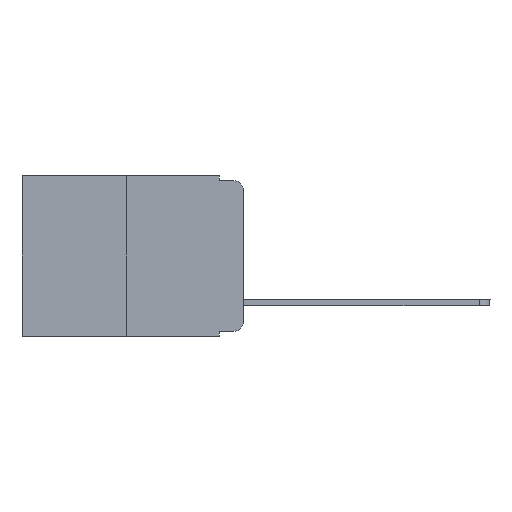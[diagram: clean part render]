
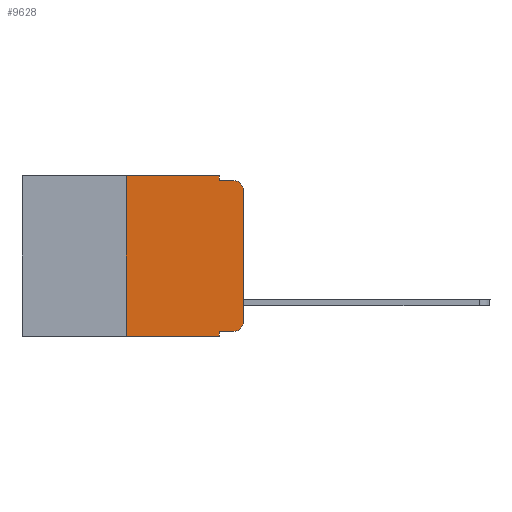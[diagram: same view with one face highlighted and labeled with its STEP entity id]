
A CAD part, left-side view. The second image highlights one B-rep face of the part: STEP entity #9628.
In plain terms, the highlighted planar face has unit normal (-1, 0, 0).
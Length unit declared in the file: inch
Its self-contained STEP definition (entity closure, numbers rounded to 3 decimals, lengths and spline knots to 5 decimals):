
#11 = EDGE_CURVE ( 'NONE', #8862, #13392, #11300, .T. ) ;
#152 = ORIENTED_EDGE ( 'NONE', *, *, #3422, .T. ) ;
#345 = EDGE_CURVE ( 'NONE', #2818, #1427, #13647, .T. ) ;
#547 = VERTEX_POINT ( 'NONE', #5646 ) ;
#638 = CARTESIAN_POINT ( 'NONE',  ( 0., 0.051, 0. ) ) ;
#684 = ORIENTED_EDGE ( 'NONE', *, *, #10073, .T. ) ;
#1288 = CARTESIAN_POINT ( 'NONE',  ( 0., 0.02, -0.01 ) ) ;
#1396 = CARTESIAN_POINT ( 'NONE',  ( 0., 0.473, 0. ) ) ;
#1427 = VERTEX_POINT ( 'NONE', #15329 ) ;
#1545 = LINE ( 'NONE', #8489, #10882 ) ;
#1700 = DIRECTION ( 'NONE',  ( 0., 0., -1. ) ) ;
#1872 = EDGE_CURVE ( 'NONE', #8344, #1427, #16747, .T. ) ;
#2056 = ORIENTED_EDGE ( 'NONE', *, *, #18135, .F. ) ;
#2408 = VECTOR ( 'NONE', #17704, 39.37008 ) ;
#2818 = VERTEX_POINT ( 'NONE', #18483 ) ;
#3417 = VERTEX_POINT ( 'NONE', #4637 ) ;
#3422 = EDGE_CURVE ( 'NONE', #17371, #13392, #4702, .T. ) ;
#3430 = ORIENTED_EDGE ( 'NONE', *, *, #345, .F. ) ;
#3858 = AXIS2_PLACEMENT_3D ( 'NONE', #16338, #9011, #1700 ) ;
#3908 = EDGE_LOOP ( 'NONE', ( #684, #152, #14595, #10687, #2056, #16641, #16863, #3430, #11222, #4939 ) ) ;
#4246 = DIRECTION ( 'NONE',  ( 0., 0., -1. ) ) ;
#4488 = DIRECTION ( 'NONE',  ( 0., -1., 0. ) ) ;
#4637 = CARTESIAN_POINT ( 'NONE',  ( 0., 0., -0.313 ) ) ;
#4702 = CIRCLE ( 'NONE', #11975, 0.02 ) ;
#4939 = ORIENTED_EDGE ( 'NONE', *, *, #8676, .T. ) ;
#5646 = CARTESIAN_POINT ( 'NONE',  ( 0., 0.051, 0. ) ) ;
#5827 = CARTESIAN_POINT ( 'NONE',  ( 0., 0.25, 0. ) ) ;
#6082 = CARTESIAN_POINT ( 'NONE',  ( 0., 0., 0. ) ) ;
#6829 = DIRECTION ( 'NONE',  ( 0., -1., 0. ) ) ;
#6892 = LINE ( 'NONE', #1396, #10741 ) ;
#7081 = DIRECTION ( 'NONE',  ( 1., 0., 0. ) ) ;
#7203 = DIRECTION ( 'NONE',  ( -1., 0., 0. ) ) ;
#7358 = DIRECTION ( 'NONE',  ( 0., -1., 0. ) ) ;
#7393 = DIRECTION ( 'NONE',  ( 0., 0., -1. ) ) ;
#7882 = DIRECTION ( 'NONE',  ( 0., -1., 0. ) ) ;
#8344 = VERTEX_POINT ( 'NONE', #14053 ) ;
#8489 = CARTESIAN_POINT ( 'NONE',  ( 0., 0.25, 0. ) ) ;
#8500 = CARTESIAN_POINT ( 'NONE',  ( 0., 0.051, -0.333 ) ) ;
#8676 = EDGE_CURVE ( 'NONE', #11493, #3417, #10803, .T. ) ;
#8687 = LINE ( 'NONE', #8500, #14367 ) ;
#8862 = VERTEX_POINT ( 'NONE', #18714 ) ;
#8868 = DIRECTION ( 'NONE',  ( 0., 0., -1. ) ) ;
#9011 = DIRECTION ( 'NONE',  ( -1., 0., 0. ) ) ;
#9628 = ADVANCED_FACE ( 'NONE', ( #17096 ), #12626, .F. ) ;
#9953 = EDGE_CURVE ( 'NONE', #8344, #13545, #1545, .T. ) ;
#10073 = EDGE_CURVE ( 'NONE', #3417, #17371, #16096, .T. ) ;
#10609 = DIRECTION ( 'NONE',  ( 0., 0., -1. ) ) ;
#10636 = CARTESIAN_POINT ( 'NONE',  ( 0., 0., -0.03 ) ) ;
#10687 = ORIENTED_EDGE ( 'NONE', *, *, #15321, .F. ) ;
#10741 = VECTOR ( 'NONE', #7358, 39.37008 ) ;
#10803 = CIRCLE ( 'NONE', #3858, 0.02 ) ;
#10882 = VECTOR ( 'NONE', #14365, 39.37008 ) ;
#11117 = CARTESIAN_POINT ( 'NONE',  ( 0., 0.051, -0.01 ) ) ;
#11222 = ORIENTED_EDGE ( 'NONE', *, *, #16514, .T. ) ;
#11300 = LINE ( 'NONE', #11117, #15533 ) ;
#11493 = VERTEX_POINT ( 'NONE', #12011 ) ;
#11520 = VECTOR ( 'NONE', #7882, 39.37008 ) ;
#11975 = AXIS2_PLACEMENT_3D ( 'NONE', #15979, #7203, #7393 ) ;
#11994 = LINE ( 'NONE', #17798, #12547 ) ;
#12011 = CARTESIAN_POINT ( 'NONE',  ( 0., 0.02, -0.333 ) ) ;
#12173 = CARTESIAN_POINT ( 'NONE',  ( 0., 0.473, -0.343 ) ) ;
#12547 = VECTOR ( 'NONE', #8868, 39.37008 ) ;
#12626 = PLANE ( 'NONE',  #17261 ) ;
#12822 = VECTOR ( 'NONE', #10609, 39.37008 ) ;
#13392 = VERTEX_POINT ( 'NONE', #1288 ) ;
#13545 = VERTEX_POINT ( 'NONE', #5827 ) ;
#13647 = LINE ( 'NONE', #638, #12822 ) ;
#14053 = CARTESIAN_POINT ( 'NONE',  ( 0., 0.25, -0.343 ) ) ;
#14365 = DIRECTION ( 'NONE',  ( 0., 0., 1. ) ) ;
#14367 = VECTOR ( 'NONE', #4488, 39.37008 ) ;
#14595 = ORIENTED_EDGE ( 'NONE', *, *, #11, .F. ) ;
#15321 = EDGE_CURVE ( 'NONE', #547, #8862, #11994, .T. ) ;
#15329 = CARTESIAN_POINT ( 'NONE',  ( 0., 0.051, -0.343 ) ) ;
#15533 = VECTOR ( 'NONE', #6829, 39.37008 ) ;
#15979 = CARTESIAN_POINT ( 'NONE',  ( 0., 0.02, -0.03 ) ) ;
#16096 = LINE ( 'NONE', #6082, #2408 ) ;
#16338 = CARTESIAN_POINT ( 'NONE',  ( 0., 0.02, -0.313 ) ) ;
#16514 = EDGE_CURVE ( 'NONE', #2818, #11493, #8687, .T. ) ;
#16641 = ORIENTED_EDGE ( 'NONE', *, *, #9953, .F. ) ;
#16747 = LINE ( 'NONE', #12173, #11520 ) ;
#16863 = ORIENTED_EDGE ( 'NONE', *, *, #1872, .T. ) ;
#17096 = FACE_OUTER_BOUND ( 'NONE', #3908, .T. ) ;
#17261 = AXIS2_PLACEMENT_3D ( 'NONE', #18434, #7081, #4246 ) ;
#17371 = VERTEX_POINT ( 'NONE', #10636 ) ;
#17704 = DIRECTION ( 'NONE',  ( 0., 0., 1. ) ) ;
#17798 = CARTESIAN_POINT ( 'NONE',  ( 0., 0.051, 0. ) ) ;
#18135 = EDGE_CURVE ( 'NONE', #13545, #547, #6892, .T. ) ;
#18434 = CARTESIAN_POINT ( 'NONE',  ( 0., 0.473, 0. ) ) ;
#18483 = CARTESIAN_POINT ( 'NONE',  ( 0., 0.051, -0.333 ) ) ;
#18714 = CARTESIAN_POINT ( 'NONE',  ( 0., 0.051, -0.01 ) ) ;
